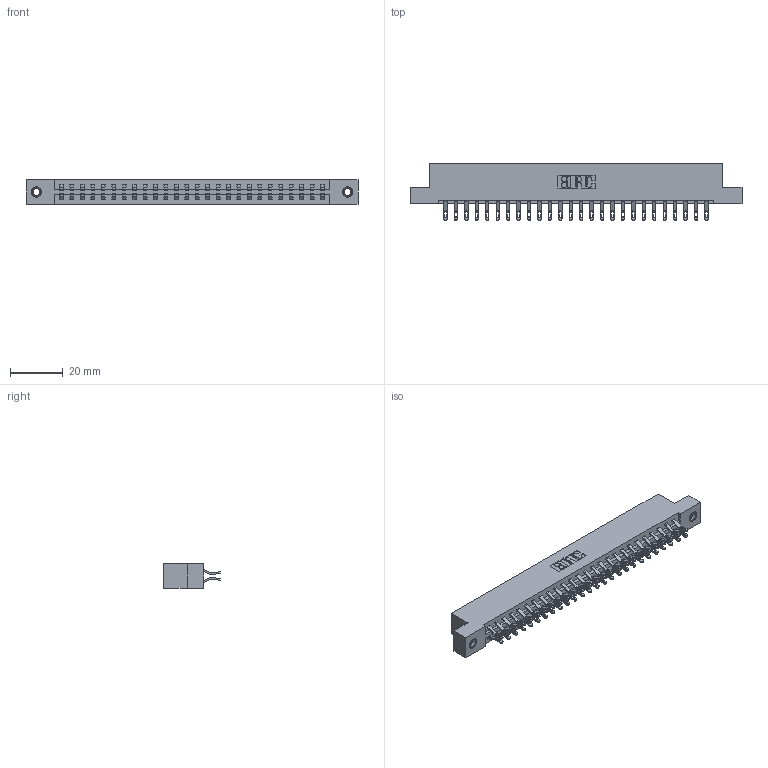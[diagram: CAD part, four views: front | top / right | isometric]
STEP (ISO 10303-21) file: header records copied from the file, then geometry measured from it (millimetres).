
FILE_DESCRIPTION (( 'STEP AP203' ), '1' );
FILE_NAME ('387-052-555-207.STEP', '2018-09-20T21:14:58', ( '' ), ( '' ), 'SwSTEP 2.0', 'SolidWorks 2016', '' );
FILE_SCHEMA (( 'CONFIG_CONTROL_DESIGN' ));
Length unit declared in the file: inch
Products named in the file (4): 337 Part_Flush Mounting Lugs - 0.156 Dia-TI; 345-292-001_555 Tail; 345-250-001_345-250-005-103; 387-052-555-207
Assembly tree (55 placements, depth 2):
  387-052-555-207
    337 Part_Flush Mounting Lugs - 0.156 Dia-TI
    345-292-001_555 Tail  x52
    345-250-001_345-250-005-103  x2
Bounding box: 126.03 x 21.47 x 9.4 mm (x, y, z)
Volume: 13206.9 mm3; surface area: 15379.3 mm2
Topology: 55 solids, 55 shells, 3294 faces, 10275 edges, 6842 vertices
Faces by surface type: plane 1974, cylinder 1304, cone 12, torus 4
Entity records: 23740 total; most frequent: CARTESIAN_POINT 4027, ORIENTED_EDGE 3926, DIRECTION 3457, EDGE_CURVE 1963, LINE 1795, VECTOR 1795, VERTEX_POINT 1304, AXIS2_PLACEMENT_3D 831
